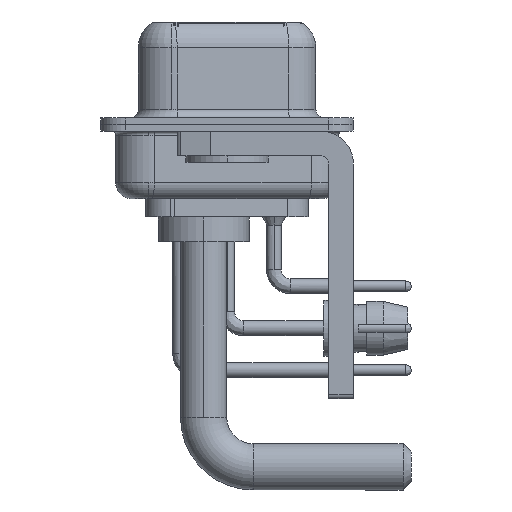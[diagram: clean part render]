
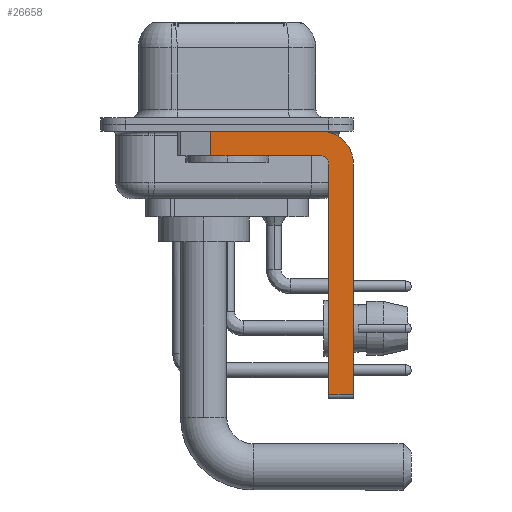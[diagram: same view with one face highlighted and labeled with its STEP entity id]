
A CAD part, left-side view. The second image highlights one B-rep face of the part: STEP entity #26658.
In plain terms, the highlighted planar face has unit normal (-1, 0, 0).
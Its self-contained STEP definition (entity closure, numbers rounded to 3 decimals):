
#149 = CARTESIAN_POINT ( 'NONE',  ( -2.9, 0.978, -1.9 ) ) ;
#698 = LINE ( 'NONE', #11454, #22721 ) ;
#1005 = EDGE_CURVE ( 'NONE', #12225, #26401, #3910, .T. ) ;
#1441 = CARTESIAN_POINT ( 'NONE',  ( -2.9, -6.15, -16.6 ) ) ;
#1793 = DIRECTION ( 'NONE',  ( 0., 0., 1. ) ) ;
#2119 = AXIS2_PLACEMENT_3D ( 'NONE', #7930, #2443, #10555 ) ;
#2408 = CARTESIAN_POINT ( 'NONE',  ( -2.9, -6.15, -2.4 ) ) ;
#2412 = VERTEX_POINT ( 'NONE', #25344 ) ;
#2443 = DIRECTION ( 'NONE',  ( 1., 0., 0. ) ) ;
#2935 = VECTOR ( 'NONE', #7746, 1000. ) ;
#3117 = EDGE_CURVE ( 'NONE', #2412, #21025, #7392, .T. ) ;
#3910 = LINE ( 'NONE', #1441, #19075 ) ;
#4192 = ORIENTED_EDGE ( 'NONE', *, *, #33278, .F. ) ;
#5801 = ORIENTED_EDGE ( 'NONE', *, *, #29091, .F. ) ;
#5935 = DIRECTION ( 'NONE',  ( 1., 0., 0. ) ) ;
#6773 = CARTESIAN_POINT ( 'NONE',  ( -2.9, -7.65, -2.4 ) ) ;
#7392 = LINE ( 'NONE', #149, #2935 ) ;
#7488 = ORIENTED_EDGE ( 'NONE', *, *, #8088, .F. ) ;
#7746 = DIRECTION ( 'NONE',  ( 0., 0., -1. ) ) ;
#7906 = DIRECTION ( 'NONE',  ( 0., 0., 1. ) ) ;
#7930 = CARTESIAN_POINT ( 'NONE',  ( -2.9, -5.65, -2.4 ) ) ;
#8088 = EDGE_CURVE ( 'NONE', #2412, #15501, #28372, .T. ) ;
#8163 = ORIENTED_EDGE ( 'NONE', *, *, #1005, .F. ) ;
#8592 = FACE_OUTER_BOUND ( 'NONE', #23748, .T. ) ;
#8866 = AXIS2_PLACEMENT_3D ( 'NONE', #26450, #10189, #7906 ) ;
#10189 = DIRECTION ( 'NONE',  ( -1., 0., 0. ) ) ;
#10555 = DIRECTION ( 'NONE',  ( 0., 0., -1. ) ) ;
#11096 = EDGE_CURVE ( 'NONE', #17038, #32531, #32472, .T. ) ;
#11454 = CARTESIAN_POINT ( 'NONE',  ( -2.9, -5.65, -16.35 ) ) ;
#12076 = LINE ( 'NONE', #32927, #29950 ) ;
#12225 = VERTEX_POINT ( 'NONE', #34787 ) ;
#12304 = CARTESIAN_POINT ( 'NONE',  ( -2.9, 3., -0.4 ) ) ;
#13899 = EDGE_CURVE ( 'NONE', #26401, #28765, #31358, .T. ) ;
#15501 = VERTEX_POINT ( 'NONE', #21804 ) ;
#15656 = CARTESIAN_POINT ( 'NONE',  ( -2.9, 0.978, -1.9 ) ) ;
#16687 = DIRECTION ( 'NONE',  ( 0., 0., -1. ) ) ;
#17038 = VERTEX_POINT ( 'NONE', #6773 ) ;
#17615 = CARTESIAN_POINT ( 'NONE',  ( -2.9, -7.65, -16.35 ) ) ;
#17823 = ORIENTED_EDGE ( 'NONE', *, *, #13899, .F. ) ;
#18018 = EDGE_CURVE ( 'NONE', #12225, #32531, #698, .T. ) ;
#18095 = AXIS2_PLACEMENT_3D ( 'NONE', #30124, #5935, #16687 ) ;
#19075 = VECTOR ( 'NONE', #1793, 1000. ) ;
#19363 = PLANE ( 'NONE',  #18095 ) ;
#20391 = VECTOR ( 'NONE', #23617, 1000. ) ;
#21025 = VERTEX_POINT ( 'NONE', #15656 ) ;
#21083 = ORIENTED_EDGE ( 'NONE', *, *, #11096, .F. ) ;
#21804 = CARTESIAN_POINT ( 'NONE',  ( -2.9, -5.65, -0.4 ) ) ;
#22245 = DIRECTION ( 'NONE',  ( 0., -1., 0. ) ) ;
#22721 = VECTOR ( 'NONE', #22245, 1000. ) ;
#22863 = DIRECTION ( 'NONE',  ( 0., 1., 0. ) ) ;
#23617 = DIRECTION ( 'NONE',  ( 0., -1., 0. ) ) ;
#23748 = EDGE_LOOP ( 'NONE', ( #7488, #31976, #4192, #17823, #8163, #30893, #21083, #5801 ) ) ;
#25344 = CARTESIAN_POINT ( 'NONE',  ( -2.9, 0.978, -0.4 ) ) ;
#26401 = VERTEX_POINT ( 'NONE', #2408 ) ;
#26450 = CARTESIAN_POINT ( 'NONE',  ( -2.9, -5.65, -2.4 ) ) ;
#26658 = ADVANCED_FACE ( 'NONE', ( #8592 ), #19363, .F. ) ;
#28372 = LINE ( 'NONE', #12304, #20391 ) ;
#28765 = VERTEX_POINT ( 'NONE', #29858 ) ;
#29091 = EDGE_CURVE ( 'NONE', #15501, #17038, #33699, .T. ) ;
#29858 = CARTESIAN_POINT ( 'NONE',  ( -2.9, -5.65, -1.9 ) ) ;
#29950 = VECTOR ( 'NONE', #22863, 1000. ) ;
#30124 = CARTESIAN_POINT ( 'NONE',  ( -2.9, -5.65, -2.4 ) ) ;
#30893 = ORIENTED_EDGE ( 'NONE', *, *, #18018, .T. ) ;
#31358 = CIRCLE ( 'NONE', #8866, 0.5 ) ;
#31976 = ORIENTED_EDGE ( 'NONE', *, *, #3117, .T. ) ;
#32472 = LINE ( 'NONE', #32661, #33004 ) ;
#32531 = VERTEX_POINT ( 'NONE', #17615 ) ;
#32661 = CARTESIAN_POINT ( 'NONE',  ( -2.9, -7.65, -2.4 ) ) ;
#32927 = CARTESIAN_POINT ( 'NONE',  ( -2.9, -5.65, -1.9 ) ) ;
#33002 = DIRECTION ( 'NONE',  ( 0., 0., -1. ) ) ;
#33004 = VECTOR ( 'NONE', #33002, 1000. ) ;
#33278 = EDGE_CURVE ( 'NONE', #28765, #21025, #12076, .T. ) ;
#33699 = CIRCLE ( 'NONE', #2119, 2. ) ;
#34787 = CARTESIAN_POINT ( 'NONE',  ( -2.9, -6.15, -16.35 ) ) ;
